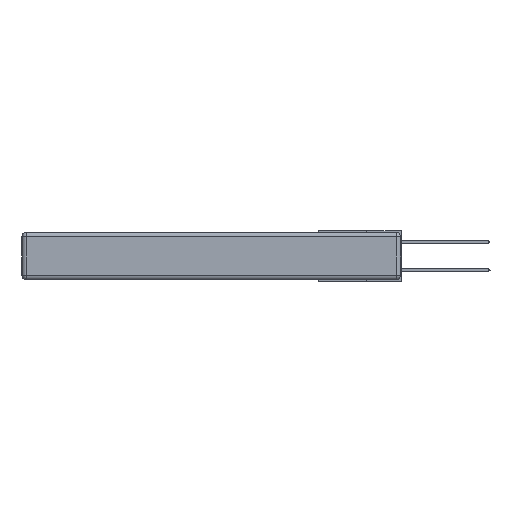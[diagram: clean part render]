
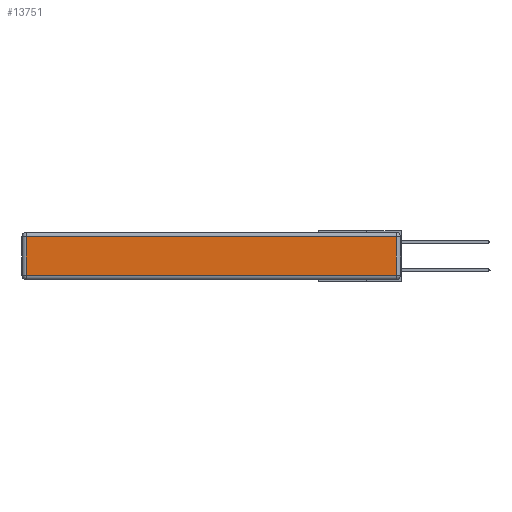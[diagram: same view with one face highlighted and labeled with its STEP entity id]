
A CAD part, left-side view. The second image highlights one B-rep face of the part: STEP entity #13751.
In plain terms, the highlighted planar face has unit normal (-1, 0, 0).
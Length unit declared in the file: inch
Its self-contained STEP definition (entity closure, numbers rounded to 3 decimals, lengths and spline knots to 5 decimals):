
#952 = VECTOR ( 'NONE', #27599, 39.37008 ) ;
#1779 = LINE ( 'NONE', #2914, #952 ) ;
#2289 = VERTEX_POINT ( 'NONE', #28495 ) ;
#2473 = CARTESIAN_POINT ( 'NONE',  ( 0., 0.03, -0.03 ) ) ;
#2914 = CARTESIAN_POINT ( 'NONE',  ( 0., 0., -0.313 ) ) ;
#4328 = DIRECTION ( 'NONE',  ( -1., 0., 0. ) ) ;
#10707 = EDGE_LOOP ( 'NONE', ( #34798, #29330, #24024, #24586 ) ) ;
#11877 = CARTESIAN_POINT ( 'NONE',  ( 0., 0.03, -0.343 ) ) ;
#13645 = VERTEX_POINT ( 'NONE', #33552 ) ;
#13751 = ADVANCED_FACE ( 'NONE', ( #23843 ), #26476, .T. ) ;
#13826 = VECTOR ( 'NONE', #24081, 39.37008 ) ;
#16954 = VECTOR ( 'NONE', #25860, 39.37008 ) ;
#17412 = CARTESIAN_POINT ( 'NONE',  ( 0., 2.72, -0.03 ) ) ;
#17860 = VECTOR ( 'NONE', #19139, 39.37008 ) ;
#18393 = EDGE_CURVE ( 'NONE', #31879, #20489, #25267, .T. ) ;
#19139 = DIRECTION ( 'NONE',  ( 0., 1., 0. ) ) ;
#20200 = AXIS2_PLACEMENT_3D ( 'NONE', #34869, #4328, #34985 ) ;
#20489 = VERTEX_POINT ( 'NONE', #17412 ) ;
#21292 = EDGE_CURVE ( 'NONE', #13645, #2289, #1779, .T. ) ;
#22950 = CARTESIAN_POINT ( 'NONE',  ( 0., 2.72, -0.343 ) ) ;
#23843 = FACE_OUTER_BOUND ( 'NONE', #10707, .T. ) ;
#24024 = ORIENTED_EDGE ( 'NONE', *, *, #18393, .T. ) ;
#24081 = DIRECTION ( 'NONE',  ( 0., 0., -1. ) ) ;
#24586 = ORIENTED_EDGE ( 'NONE', *, *, #33217, .T. ) ;
#25267 = LINE ( 'NONE', #35930, #17860 ) ;
#25860 = DIRECTION ( 'NONE',  ( 0., 0., 1. ) ) ;
#26476 = PLANE ( 'NONE',  #20200 ) ;
#27599 = DIRECTION ( 'NONE',  ( 0., -1., 0. ) ) ;
#27842 = LINE ( 'NONE', #11877, #16954 ) ;
#28168 = EDGE_CURVE ( 'NONE', #2289, #31879, #27842, .T. ) ;
#28495 = CARTESIAN_POINT ( 'NONE',  ( 0., 0.03, -0.313 ) ) ;
#29037 = LINE ( 'NONE', #22950, #13826 ) ;
#29330 = ORIENTED_EDGE ( 'NONE', *, *, #28168, .T. ) ;
#31879 = VERTEX_POINT ( 'NONE', #2473 ) ;
#33217 = EDGE_CURVE ( 'NONE', #20489, #13645, #29037, .T. ) ;
#33552 = CARTESIAN_POINT ( 'NONE',  ( 0., 2.72, -0.313 ) ) ;
#34798 = ORIENTED_EDGE ( 'NONE', *, *, #21292, .T. ) ;
#34869 = CARTESIAN_POINT ( 'NONE',  ( 0., 0., -0.343 ) ) ;
#34985 = DIRECTION ( 'NONE',  ( 0., 0., 1. ) ) ;
#35930 = CARTESIAN_POINT ( 'NONE',  ( 0., 2.75, -0.03 ) ) ;
